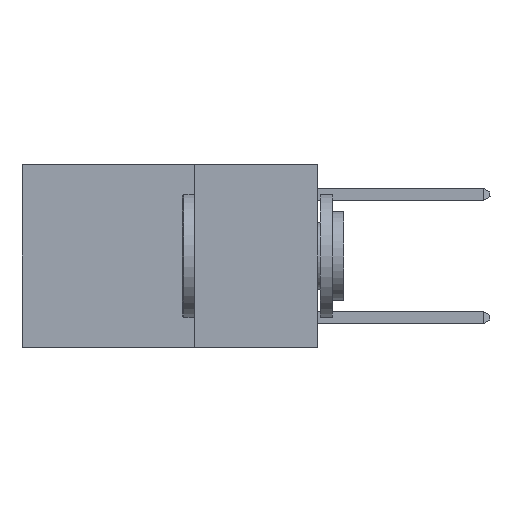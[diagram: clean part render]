
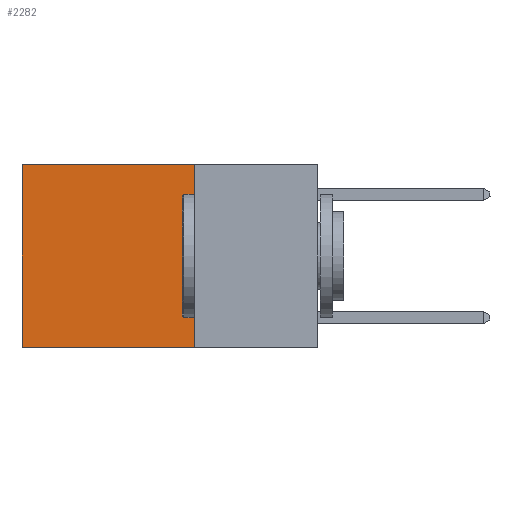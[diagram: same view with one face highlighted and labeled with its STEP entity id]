
A CAD part, left-side view. The second image highlights one B-rep face of the part: STEP entity #2282.
In plain terms, the highlighted planar face has unit normal (-1, 0, 0).
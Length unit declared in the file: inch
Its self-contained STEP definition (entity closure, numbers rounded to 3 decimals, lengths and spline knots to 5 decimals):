
#76 = CARTESIAN_POINT ( 'NONE',  ( 0.2625, 0.6, -0.37 ) ) ;
#643 = ORIENTED_EDGE ( 'NONE', *, *, #10729, .T. ) ;
#847 = ORIENTED_EDGE ( 'NONE', *, *, #8735, .T. ) ;
#901 = LINE ( 'NONE', #3764, #8649 ) ;
#1152 = CARTESIAN_POINT ( 'NONE',  ( 0.2625, 0.25, 0. ) ) ;
#2282 = ADVANCED_FACE ( 'NONE', ( #8482 ), #7057, .F. ) ;
#2485 = VECTOR ( 'NONE', #11495, 39.37008 ) ;
#3022 = CARTESIAN_POINT ( 'NONE',  ( 0.2625, 0.25, -0.37 ) ) ;
#3179 = CARTESIAN_POINT ( 'NONE',  ( 0.2625, 0.25, 0. ) ) ;
#3366 = CARTESIAN_POINT ( 'NONE',  ( 0.2625, 0.25, 0. ) ) ;
#3414 = ORIENTED_EDGE ( 'NONE', *, *, #11089, .F. ) ;
#3614 = VERTEX_POINT ( 'NONE', #3179 ) ;
#3671 = VERTEX_POINT ( 'NONE', #76 ) ;
#3764 = CARTESIAN_POINT ( 'NONE',  ( 0.2625, 0.6, 0. ) ) ;
#3981 = LINE ( 'NONE', #3366, #11031 ) ;
#4014 = ORIENTED_EDGE ( 'NONE', *, *, #11359, .F. ) ;
#4475 = VECTOR ( 'NONE', #10122, 39.37008 ) ;
#4565 = DIRECTION ( 'NONE',  ( 0., 0., -1. ) ) ;
#4668 = DIRECTION ( 'NONE',  ( 1., 0., 0. ) ) ;
#4754 = VERTEX_POINT ( 'NONE', #6015 ) ;
#5697 = CARTESIAN_POINT ( 'NONE',  ( 0.2625, 0.25, 0. ) ) ;
#6015 = CARTESIAN_POINT ( 'NONE',  ( 0.2625, 0.6, 0. ) ) ;
#6377 = EDGE_LOOP ( 'NONE', ( #847, #3414, #4014, #643 ) ) ;
#6937 = VERTEX_POINT ( 'NONE', #3022 ) ;
#7057 = PLANE ( 'NONE',  #7888 ) ;
#7138 = LINE ( 'NONE', #1152, #4475 ) ;
#7888 = AXIS2_PLACEMENT_3D ( 'NONE', #5697, #4668, #4565 ) ;
#8482 = FACE_OUTER_BOUND ( 'NONE', #6377, .T. ) ;
#8649 = VECTOR ( 'NONE', #10561, 39.37008 ) ;
#8735 = EDGE_CURVE ( 'NONE', #4754, #3671, #901, .T. ) ;
#8842 = CARTESIAN_POINT ( 'NONE',  ( 0.2625, 0.25, -0.37 ) ) ;
#9264 = DIRECTION ( 'NONE',  ( 0., 1., 0. ) ) ;
#10053 = LINE ( 'NONE', #8842, #2485 ) ;
#10122 = DIRECTION ( 'NONE',  ( 0., 0., -1. ) ) ;
#10561 = DIRECTION ( 'NONE',  ( 0., 0., -1. ) ) ;
#10729 = EDGE_CURVE ( 'NONE', #3614, #4754, #3981, .T. ) ;
#11031 = VECTOR ( 'NONE', #9264, 39.37008 ) ;
#11089 = EDGE_CURVE ( 'NONE', #6937, #3671, #10053, .T. ) ;
#11359 = EDGE_CURVE ( 'NONE', #3614, #6937, #7138, .T. ) ;
#11495 = DIRECTION ( 'NONE',  ( 0., 1., 0. ) ) ;
